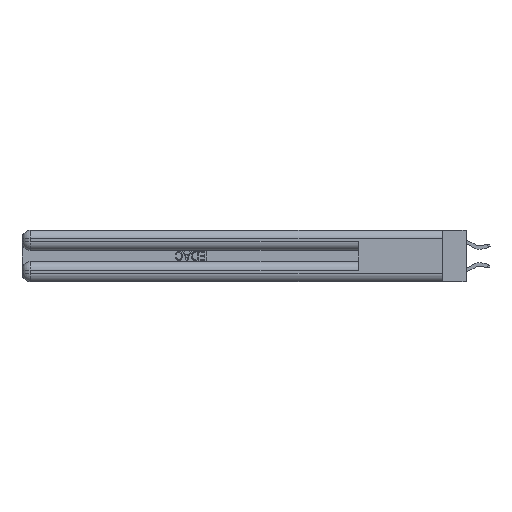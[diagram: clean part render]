
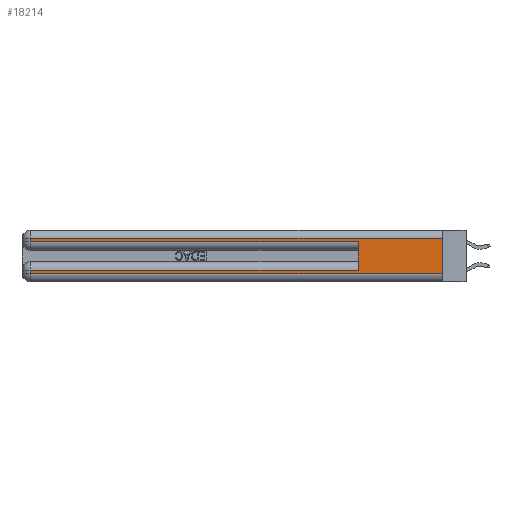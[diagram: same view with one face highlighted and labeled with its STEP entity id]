
A CAD part, left-side view. The second image highlights one B-rep face of the part: STEP entity #18214.
In plain terms, the highlighted planar face has unit normal (-1, 0, 0).
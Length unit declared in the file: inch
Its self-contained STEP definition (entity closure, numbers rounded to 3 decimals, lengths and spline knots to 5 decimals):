
#1546 = CARTESIAN_POINT ( 'NONE',  ( 0., 0., 0.31 ) ) ;
#1567 = VECTOR ( 'NONE', #10689, 39.37008 ) ;
#2579 = DIRECTION ( 'NONE',  ( 0., 0., -1. ) ) ;
#2710 = ORIENTED_EDGE ( 'NONE', *, *, #17678, .F. ) ;
#3331 = LINE ( 'NONE', #20826, #31253 ) ;
#4329 = LINE ( 'NONE', #22101, #26096 ) ;
#4520 = CARTESIAN_POINT ( 'NONE',  ( 0., 2.94, 0.285 ) ) ;
#4527 = PLANE ( 'NONE',  #6625 ) ;
#4712 = EDGE_CURVE ( 'NONE', #9844, #7899, #25608, .T. ) ;
#4789 = DIRECTION ( 'NONE',  ( 0., 0., 1. ) ) ;
#4950 = DIRECTION ( 'NONE',  ( 0., 0., -1. ) ) ;
#5160 = VERTEX_POINT ( 'NONE', #19596 ) ;
#5674 = LINE ( 'NONE', #1546, #32778 ) ;
#6625 = AXIS2_PLACEMENT_3D ( 'NONE', #28176, #12455, #30797 ) ;
#7808 = VERTEX_POINT ( 'NONE', #22523 ) ;
#7899 = VERTEX_POINT ( 'NONE', #15066 ) ;
#8526 = EDGE_CURVE ( 'NONE', #5160, #14050, #5674, .T. ) ;
#8591 = LINE ( 'NONE', #29046, #1567 ) ;
#8844 = CARTESIAN_POINT ( 'NONE',  ( 0., 2.94, 0.31 ) ) ;
#8954 = EDGE_CURVE ( 'NONE', #9844, #18744, #27911, .T. ) ;
#9844 = VERTEX_POINT ( 'NONE', #12532 ) ;
#10689 = DIRECTION ( 'NONE',  ( 0., 0., -1. ) ) ;
#11199 = CARTESIAN_POINT ( 'NONE',  ( 0., 0., 0.085 ) ) ;
#11264 = ORIENTED_EDGE ( 'NONE', *, *, #18910, .T. ) ;
#11671 = CARTESIAN_POINT ( 'NONE',  ( 0., 0., 0.06 ) ) ;
#12455 = DIRECTION ( 'NONE',  ( 1., 0., 0. ) ) ;
#12532 = CARTESIAN_POINT ( 'NONE',  ( 0., 0.6, 0.085 ) ) ;
#14050 = VERTEX_POINT ( 'NONE', #8844 ) ;
#14051 = ORIENTED_EDGE ( 'NONE', *, *, #4712, .F. ) ;
#14313 = DIRECTION ( 'NONE',  ( 0., -1., 0. ) ) ;
#14786 = EDGE_CURVE ( 'NONE', #29418, #7899, #4329, .T. ) ;
#14791 = EDGE_CURVE ( 'NONE', #19712, #7808, #32221, .T. ) ;
#15029 = DIRECTION ( 'NONE',  ( 0., 1., 0. ) ) ;
#15066 = CARTESIAN_POINT ( 'NONE',  ( 0., 0.6, 0.285 ) ) ;
#16841 = DIRECTION ( 'NONE',  ( 0., -1., 0. ) ) ;
#17493 = VECTOR ( 'NONE', #14313, 39.37008 ) ;
#17678 = EDGE_CURVE ( 'NONE', #5160, #7808, #23838, .T. ) ;
#17681 = ORIENTED_EDGE ( 'NONE', *, *, #8954, .T. ) ;
#17820 = VECTOR ( 'NONE', #4789, 39.37008 ) ;
#17909 = CARTESIAN_POINT ( 'NONE',  ( 0., 0.6, 0.145 ) ) ;
#18214 = ADVANCED_FACE ( 'NONE', ( #29120 ), #4527, .F. ) ;
#18345 = CARTESIAN_POINT ( 'NONE',  ( 0., 0., 0.37 ) ) ;
#18386 = ORIENTED_EDGE ( 'NONE', *, *, #14791, .T. ) ;
#18744 = VERTEX_POINT ( 'NONE', #23228 ) ;
#18910 = EDGE_CURVE ( 'NONE', #18744, #19712, #8591, .T. ) ;
#19596 = CARTESIAN_POINT ( 'NONE',  ( 0., 0., 0.31 ) ) ;
#19712 = VERTEX_POINT ( 'NONE', #24308 ) ;
#20826 = CARTESIAN_POINT ( 'NONE',  ( 0., 2.94, 0.37 ) ) ;
#20944 = VECTOR ( 'NONE', #32165, 39.37008 ) ;
#22101 = CARTESIAN_POINT ( 'NONE',  ( 0., 0., 0.285 ) ) ;
#22523 = CARTESIAN_POINT ( 'NONE',  ( 0., 0., 0.06 ) ) ;
#22978 = ORIENTED_EDGE ( 'NONE', *, *, #14786, .T. ) ;
#23228 = CARTESIAN_POINT ( 'NONE',  ( 0., 2.94, 0.085 ) ) ;
#23838 = LINE ( 'NONE', #18345, #25500 ) ;
#24308 = CARTESIAN_POINT ( 'NONE',  ( 0., 2.94, 0.06 ) ) ;
#25495 = ORIENTED_EDGE ( 'NONE', *, *, #8526, .T. ) ;
#25500 = VECTOR ( 'NONE', #2579, 39.37008 ) ;
#25608 = LINE ( 'NONE', #17909, #17820 ) ;
#25675 = EDGE_LOOP ( 'NONE', ( #2710, #25495, #31728, #22978, #14051, #17681, #11264, #18386 ) ) ;
#26096 = VECTOR ( 'NONE', #16841, 39.37008 ) ;
#27911 = LINE ( 'NONE', #11199, #20944 ) ;
#28176 = CARTESIAN_POINT ( 'NONE',  ( 0., 0., 0.37 ) ) ;
#29046 = CARTESIAN_POINT ( 'NONE',  ( 0., 2.94, 0.37 ) ) ;
#29120 = FACE_OUTER_BOUND ( 'NONE', #25675, .T. ) ;
#29418 = VERTEX_POINT ( 'NONE', #4520 ) ;
#30797 = DIRECTION ( 'NONE',  ( 0., 0., -1. ) ) ;
#31253 = VECTOR ( 'NONE', #4950, 39.37008 ) ;
#31613 = EDGE_CURVE ( 'NONE', #14050, #29418, #3331, .T. ) ;
#31728 = ORIENTED_EDGE ( 'NONE', *, *, #31613, .T. ) ;
#32165 = DIRECTION ( 'NONE',  ( 0., 1., 0. ) ) ;
#32221 = LINE ( 'NONE', #11671, #17493 ) ;
#32778 = VECTOR ( 'NONE', #15029, 39.37008 ) ;
